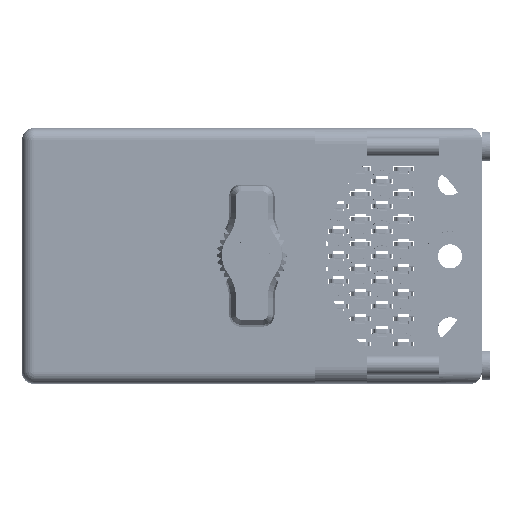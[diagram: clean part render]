
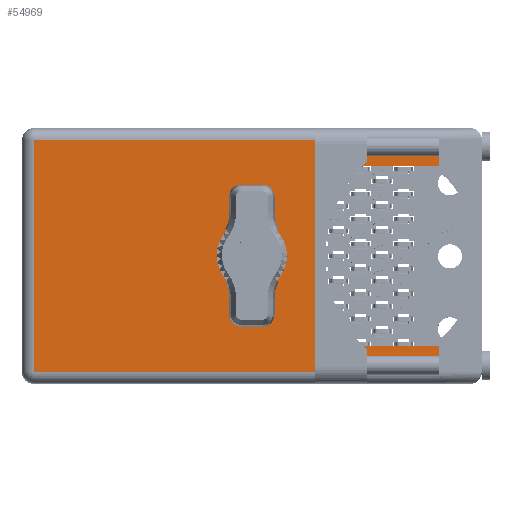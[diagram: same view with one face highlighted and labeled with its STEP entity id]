
A CAD part, top view. The second image highlights one B-rep face of the part: STEP entity #54969.
In plain terms, the highlighted face is planar.
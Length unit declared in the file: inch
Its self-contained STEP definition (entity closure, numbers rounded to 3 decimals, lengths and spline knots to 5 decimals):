
#462 = LINE ( 'NONE', #17533, #101893 ) ;
#2512 = VECTOR ( 'NONE', #15254, 39.37008 ) ;
#2582 = LINE ( 'NONE', #99895, #64356 ) ;
#3742 = ORIENTED_EDGE ( 'NONE', *, *, #101525, .T. ) ;
#6516 = CARTESIAN_POINT ( 'NONE',  ( -1.3075, 1.93, 0.695 ) ) ;
#7019 = DIRECTION ( 'NONE',  ( 0., 0., 1. ) ) ;
#8706 = DIRECTION ( 'NONE',  ( 0., 0., 1. ) ) ;
#9285 = VERTEX_POINT ( 'NONE', #52197 ) ;
#10371 = CARTESIAN_POINT ( 'NONE',  ( 1.1215, 1.93, 0.54 ) ) ;
#10536 = CARTESIAN_POINT ( 'NONE',  ( -1.3775, 1.93, -0.765 ) ) ;
#10593 = CARTESIAN_POINT ( 'NONE',  ( 0., 1.93, 0. ) ) ;
#11275 = EDGE_CURVE ( 'NONE', #50449, #13373, #462, .T. ) ;
#13373 = VERTEX_POINT ( 'NONE', #18753 ) ;
#15254 = DIRECTION ( 'NONE',  ( 1., 0., 0. ) ) ;
#15491 = CARTESIAN_POINT ( 'NONE',  ( 1.1215, 1.93, -0.695 ) ) ;
#15683 = CARTESIAN_POINT ( 'NONE',  ( 1.1215, 1.93, 0.54 ) ) ;
#17352 = LINE ( 'NONE', #99706, #87697 ) ;
#17533 = CARTESIAN_POINT ( 'NONE',  ( 1.1215, 1.93, -0.765 ) ) ;
#17946 = EDGE_CURVE ( 'NONE', #84509, #35919, #99336, .T. ) ;
#18753 = CARTESIAN_POINT ( 'NONE',  ( 1.1215, 1.93, 0.695 ) ) ;
#20307 = AXIS2_PLACEMENT_3D ( 'NONE', #10593, #43232, #58711 ) ;
#22336 = ORIENTED_EDGE ( 'NONE', *, *, #25908, .T. ) ;
#22802 = EDGE_CURVE ( 'NONE', #50449, #101069, #83047, .T. ) ;
#23182 = EDGE_CURVE ( 'NONE', #77654, #76232, #2582, .T. ) ;
#23788 = VECTOR ( 'NONE', #24658, 39.37008 ) ;
#24658 = DIRECTION ( 'NONE',  ( -1., 0., 0. ) ) ;
#25029 = DIRECTION ( 'NONE',  ( 0., 0., 1. ) ) ;
#25908 = EDGE_CURVE ( 'NONE', #9285, #79424, #104458, .T. ) ;
#26129 = ORIENTED_EDGE ( 'NONE', *, *, #105022, .F. ) ;
#30496 = VECTOR ( 'NONE', #32154, 39.37008 ) ;
#30870 = ORIENTED_EDGE ( 'NONE', *, *, #102685, .T. ) ;
#31717 = CARTESIAN_POINT ( 'NONE',  ( 0., 1.93, 0. ) ) ;
#32154 = DIRECTION ( 'NONE',  ( 0., 0., 1. ) ) ;
#32712 = LINE ( 'NONE', #65331, #23788 ) ;
#35919 = VERTEX_POINT ( 'NONE', #67883 ) ;
#39253 = ORIENTED_EDGE ( 'NONE', *, *, #11275, .F. ) ;
#40622 = VECTOR ( 'NONE', #64895, 39.37008 ) ;
#40646 = CARTESIAN_POINT ( 'NONE',  ( 1.1215, 1.93, -0.54 ) ) ;
#40874 = EDGE_LOOP ( 'NONE', ( #67674, #30870, #39253, #105639, #3742, #22336, #26129, #79358 ) ) ;
#42116 = PLANE ( 'NONE',  #104239 ) ;
#43232 = DIRECTION ( 'NONE',  ( 0., 1., 0. ) ) ;
#45078 = ORIENTED_EDGE ( 'NONE', *, *, #92924, .F. ) ;
#45907 = CARTESIAN_POINT ( 'NONE',  ( 0.4075, 1.93, 0.54 ) ) ;
#47179 = CARTESIAN_POINT ( 'NONE',  ( -1.3075, 1.93, -0.695 ) ) ;
#50449 = VERTEX_POINT ( 'NONE', #10371 ) ;
#51833 = LINE ( 'NONE', #97604, #2512 ) ;
#52197 = CARTESIAN_POINT ( 'NONE',  ( 0.4075, 1.93, -0.54 ) ) ;
#53610 = CARTESIAN_POINT ( 'NONE',  ( 0., 1.93, -0.17 ) ) ;
#54969 = ADVANCED_FACE ( 'NONE', ( #84323, #99848 ), #42116, .T. ) ;
#57918 = DIRECTION ( 'NONE',  ( -1., 0., 0. ) ) ;
#58711 = DIRECTION ( 'NONE',  ( 0., 0., 1. ) ) ;
#62578 = VECTOR ( 'NONE', #57918, 39.37008 ) ;
#64356 = VECTOR ( 'NONE', #7019, 39.37008 ) ;
#64775 = CARTESIAN_POINT ( 'NONE',  ( 1.1215, 1.93, -0.765 ) ) ;
#64895 = DIRECTION ( 'NONE',  ( 1., 0., 0. ) ) ;
#65331 = CARTESIAN_POINT ( 'NONE',  ( -1.3775, 1.93, -0.695 ) ) ;
#67674 = ORIENTED_EDGE ( 'NONE', *, *, #23182, .T. ) ;
#67883 = CARTESIAN_POINT ( 'NONE',  ( 0., 1.93, 0.17 ) ) ;
#68282 = DIRECTION ( 'NONE',  ( -1., 0., 0. ) ) ;
#74621 = DIRECTION ( 'NONE',  ( 0., 0., -1. ) ) ;
#76232 = VERTEX_POINT ( 'NONE', #6516 ) ;
#77654 = VERTEX_POINT ( 'NONE', #47179 ) ;
#79358 = ORIENTED_EDGE ( 'NONE', *, *, #95326, .T. ) ;
#79424 = VERTEX_POINT ( 'NONE', #40646 ) ;
#80559 = VERTEX_POINT ( 'NONE', #15491 ) ;
#81434 = DIRECTION ( 'NONE',  ( 0., 1., 0. ) ) ;
#82318 = AXIS2_PLACEMENT_3D ( 'NONE', #31717, #81434, #8706 ) ;
#83047 = LINE ( 'NONE', #15683, #62578 ) ;
#84097 = ORIENTED_EDGE ( 'NONE', *, *, #17946, .F. ) ;
#84323 = FACE_OUTER_BOUND ( 'NONE', #40874, .T. ) ;
#84509 = VERTEX_POINT ( 'NONE', #53610 ) ;
#87697 = VECTOR ( 'NONE', #74621, 39.37008 ) ;
#91819 = DIRECTION ( 'NONE',  ( 0., 1., 0. ) ) ;
#92924 = EDGE_CURVE ( 'NONE', #35919, #84509, #98873, .T. ) ;
#95326 = EDGE_CURVE ( 'NONE', #80559, #77654, #32712, .T. ) ;
#96559 = EDGE_LOOP ( 'NONE', ( #45078, #84097 ) ) ;
#97604 = CARTESIAN_POINT ( 'NONE',  ( 1.1215, 1.93, 0.695 ) ) ;
#98873 = CIRCLE ( 'NONE', #20307, 0.17 ) ;
#99336 = CIRCLE ( 'NONE', #82318, 0.17 ) ;
#99706 = CARTESIAN_POINT ( 'NONE',  ( 0.4075, 1.93, -0.54 ) ) ;
#99848 = FACE_BOUND ( 'NONE', #96559, .T. ) ;
#99895 = CARTESIAN_POINT ( 'NONE',  ( -1.3075, 1.93, -0.765 ) ) ;
#101069 = VERTEX_POINT ( 'NONE', #45907 ) ;
#101525 = EDGE_CURVE ( 'NONE', #101069, #9285, #17352, .T. ) ;
#101893 = VECTOR ( 'NONE', #25029, 39.37008 ) ;
#102685 = EDGE_CURVE ( 'NONE', #76232, #13373, #51833, .T. ) ;
#104239 = AXIS2_PLACEMENT_3D ( 'NONE', #10536, #91819, #68282 ) ;
#104458 = LINE ( 'NONE', #105525, #40622 ) ;
#105022 = EDGE_CURVE ( 'NONE', #80559, #79424, #105403, .T. ) ;
#105403 = LINE ( 'NONE', #64775, #30496 ) ;
#105525 = CARTESIAN_POINT ( 'NONE',  ( 1.1215, 1.93, -0.54 ) ) ;
#105639 = ORIENTED_EDGE ( 'NONE', *, *, #22802, .T. ) ;
